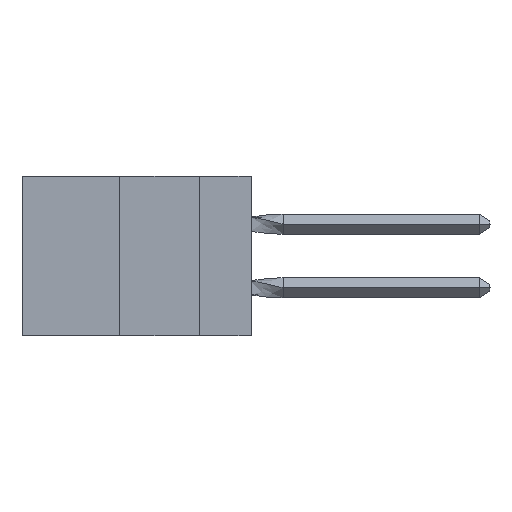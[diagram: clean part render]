
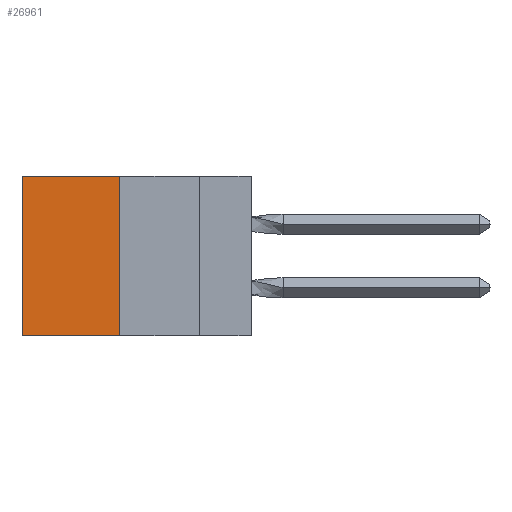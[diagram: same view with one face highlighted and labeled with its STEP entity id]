
A CAD part, left-side view. The second image highlights one B-rep face of the part: STEP entity #26961.
In plain terms, the highlighted planar face has unit normal (-1, 0, 0).
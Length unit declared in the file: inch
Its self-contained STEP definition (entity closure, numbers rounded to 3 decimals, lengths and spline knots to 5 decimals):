
#1943 = EDGE_LOOP ( 'NONE', ( #20211, #27041, #36044, #26194 ) ) ;
#2487 = DIRECTION ( 'NONE',  ( 0., 0., -1. ) ) ;
#2901 = CARTESIAN_POINT ( 'NONE',  ( 0.305, 0.72, -0.5 ) ) ;
#3714 = EDGE_CURVE ( 'NONE', #11143, #6180, #21247, .T. ) ;
#6180 = VERTEX_POINT ( 'NONE', #2901 ) ;
#7812 = EDGE_CURVE ( 'NONE', #21470, #11143, #19475, .T. ) ;
#9385 = CARTESIAN_POINT ( 'NONE',  ( 0.305, 0.413, -0.5 ) ) ;
#11143 = VERTEX_POINT ( 'NONE', #28647 ) ;
#12195 = VECTOR ( 'NONE', #2487, 39.37008 ) ;
#12896 = DIRECTION ( 'NONE',  ( 1., 0., 0. ) ) ;
#13740 = VECTOR ( 'NONE', #30453, 39.37008 ) ;
#16277 = CARTESIAN_POINT ( 'NONE',  ( 0.305, 0.413, 0. ) ) ;
#16889 = DIRECTION ( 'NONE',  ( 0., 1., 0. ) ) ;
#18376 = CARTESIAN_POINT ( 'NONE',  ( 0.305, 0.72, 0. ) ) ;
#18467 = CARTESIAN_POINT ( 'NONE',  ( 0.305, 0.72, -0.5 ) ) ;
#18715 = DIRECTION ( 'NONE',  ( 0., 1., 0. ) ) ;
#19475 = LINE ( 'NONE', #39180, #12195 ) ;
#19974 = AXIS2_PLACEMENT_3D ( 'NONE', #28252, #12896, #21894 ) ;
#20211 = ORIENTED_EDGE ( 'NONE', *, *, #26089, .T. ) ;
#21247 = LINE ( 'NONE', #9385, #35286 ) ;
#21470 = VERTEX_POINT ( 'NONE', #16277 ) ;
#21894 = DIRECTION ( 'NONE',  ( 0., 0., -1. ) ) ;
#23065 = LINE ( 'NONE', #25721, #38022 ) ;
#25267 = VERTEX_POINT ( 'NONE', #18376 ) ;
#25721 = CARTESIAN_POINT ( 'NONE',  ( 0.305, 0.413, 0. ) ) ;
#26089 = EDGE_CURVE ( 'NONE', #25267, #6180, #38314, .T. ) ;
#26194 = ORIENTED_EDGE ( 'NONE', *, *, #30816, .T. ) ;
#26961 = ADVANCED_FACE ( 'NONE', ( #29069 ), #28102, .F. ) ;
#27041 = ORIENTED_EDGE ( 'NONE', *, *, #3714, .F. ) ;
#28102 = PLANE ( 'NONE',  #19974 ) ;
#28252 = CARTESIAN_POINT ( 'NONE',  ( 0.305, 0.413, -0.5 ) ) ;
#28647 = CARTESIAN_POINT ( 'NONE',  ( 0.305, 0.413, -0.5 ) ) ;
#29069 = FACE_OUTER_BOUND ( 'NONE', #1943, .T. ) ;
#30453 = DIRECTION ( 'NONE',  ( 0., 0., -1. ) ) ;
#30816 = EDGE_CURVE ( 'NONE', #21470, #25267, #23065, .T. ) ;
#35286 = VECTOR ( 'NONE', #18715, 39.37008 ) ;
#36044 = ORIENTED_EDGE ( 'NONE', *, *, #7812, .F. ) ;
#38022 = VECTOR ( 'NONE', #16889, 39.37008 ) ;
#38314 = LINE ( 'NONE', #18467, #13740 ) ;
#39180 = CARTESIAN_POINT ( 'NONE',  ( 0.305, 0.413, -0.5 ) ) ;
